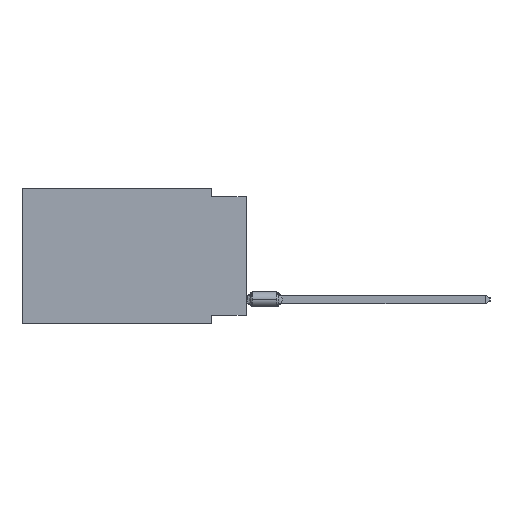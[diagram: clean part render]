
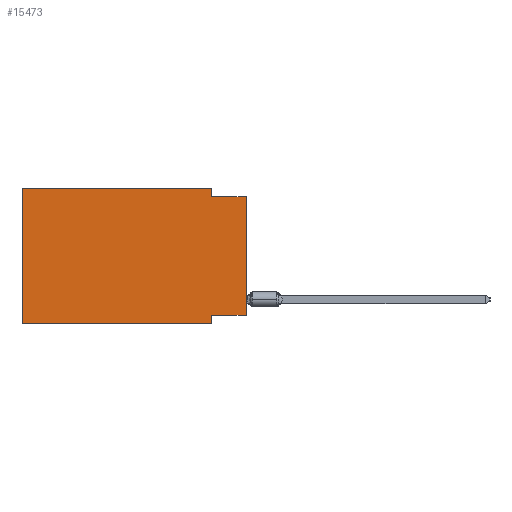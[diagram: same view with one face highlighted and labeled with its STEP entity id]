
A CAD part, left-side view. The second image highlights one B-rep face of the part: STEP entity #15473.
In plain terms, the highlighted planar face has unit normal (-1, 0, 0).
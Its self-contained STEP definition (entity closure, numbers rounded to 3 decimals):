
#1035 = DIRECTION ( 'NONE',  ( 0., -1., 0. ) ) ;
#1457 = CARTESIAN_POINT ( 'NONE',  ( 0., 0., -9.271 ) ) ;
#1651 = VECTOR ( 'NONE', #9837, 1000. ) ;
#3708 = CARTESIAN_POINT ( 'NONE',  ( 0., 2.54, 0. ) ) ;
#3875 = CARTESIAN_POINT ( 'NONE',  ( 0., 0., -9.271 ) ) ;
#4185 = EDGE_CURVE ( 'NONE', #43685, #35259, #23246, .T. ) ;
#4319 = FACE_OUTER_BOUND ( 'NONE', #26318, .T. ) ;
#5356 = EDGE_CURVE ( 'NONE', #13402, #44287, #11194, .T. ) ;
#5426 = ORIENTED_EDGE ( 'NONE', *, *, #4185, .F. ) ;
#6379 = CARTESIAN_POINT ( 'NONE',  ( 0., 0., -0.635 ) ) ;
#7292 = CARTESIAN_POINT ( 'NONE',  ( 0., 0., -0.635 ) ) ;
#7684 = EDGE_CURVE ( 'NONE', #8545, #43685, #18270, .T. ) ;
#8232 = ORIENTED_EDGE ( 'NONE', *, *, #11466, .T. ) ;
#8545 = VERTEX_POINT ( 'NONE', #31793 ) ;
#9331 = CARTESIAN_POINT ( 'NONE',  ( 0., 16.383, -9.906 ) ) ;
#9837 = DIRECTION ( 'NONE',  ( 0., -1., 0. ) ) ;
#11177 = VECTOR ( 'NONE', #12597, 1000. ) ;
#11194 = LINE ( 'NONE', #32231, #40140 ) ;
#11239 = VECTOR ( 'NONE', #1035, 1000. ) ;
#11466 = EDGE_CURVE ( 'NONE', #13402, #20700, #35704, .T. ) ;
#11579 = CARTESIAN_POINT ( 'NONE',  ( 0., 16.383, 0. ) ) ;
#12485 = ORIENTED_EDGE ( 'NONE', *, *, #7684, .F. ) ;
#12597 = DIRECTION ( 'NONE',  ( 0., 0., 1. ) ) ;
#13402 = VERTEX_POINT ( 'NONE', #9331 ) ;
#15311 = EDGE_CURVE ( 'NONE', #38041, #29236, #24675, .T. ) ;
#15473 = ADVANCED_FACE ( 'NONE', ( #4319 ), #18426, .F. ) ;
#16829 = ORIENTED_EDGE ( 'NONE', *, *, #15311, .F. ) ;
#17326 = EDGE_CURVE ( 'NONE', #38041, #35259, #40762, .T. ) ;
#18270 = LINE ( 'NONE', #3708, #45320 ) ;
#18426 = PLANE ( 'NONE',  #26439 ) ;
#18959 = CARTESIAN_POINT ( 'NONE',  ( 0., 2.54, -9.906 ) ) ;
#19021 = CARTESIAN_POINT ( 'NONE',  ( 0., 16.383, 0. ) ) ;
#19107 = CARTESIAN_POINT ( 'NONE',  ( 0., 16.383, 0. ) ) ;
#20700 = VERTEX_POINT ( 'NONE', #29949 ) ;
#22246 = LINE ( 'NONE', #19021, #34984 ) ;
#22913 = ORIENTED_EDGE ( 'NONE', *, *, #5356, .F. ) ;
#23157 = DIRECTION ( 'NONE',  ( 0., -1., 0. ) ) ;
#23246 = LINE ( 'NONE', #6379, #1651 ) ;
#23671 = CARTESIAN_POINT ( 'NONE',  ( 0., 0., 0. ) ) ;
#24661 = ORIENTED_EDGE ( 'NONE', *, *, #17326, .T. ) ;
#24675 = LINE ( 'NONE', #3875, #37514 ) ;
#26318 = EDGE_LOOP ( 'NONE', ( #24661, #5426, #12485, #37408, #22913, #8232, #43608, #16829 ) ) ;
#26439 = AXIS2_PLACEMENT_3D ( 'NONE', #19107, #33209, #35754 ) ;
#27777 = CARTESIAN_POINT ( 'NONE',  ( 0., 2.54, -9.271 ) ) ;
#29138 = LINE ( 'NONE', #18959, #42709 ) ;
#29236 = VERTEX_POINT ( 'NONE', #27777 ) ;
#29949 = CARTESIAN_POINT ( 'NONE',  ( 0., 2.54, -9.906 ) ) ;
#31396 = EDGE_CURVE ( 'NONE', #29236, #20700, #29138, .T. ) ;
#31793 = CARTESIAN_POINT ( 'NONE',  ( 0., 2.54, 0. ) ) ;
#32231 = CARTESIAN_POINT ( 'NONE',  ( 0., 16.383, 0. ) ) ;
#33209 = DIRECTION ( 'NONE',  ( 1., 0., 0. ) ) ;
#33284 = DIRECTION ( 'NONE',  ( 0., 0., -1. ) ) ;
#34984 = VECTOR ( 'NONE', #23157, 1000. ) ;
#35259 = VERTEX_POINT ( 'NONE', #7292 ) ;
#35360 = DIRECTION ( 'NONE',  ( 0., 0., -1. ) ) ;
#35689 = DIRECTION ( 'NONE',  ( 0., 0., 1. ) ) ;
#35704 = LINE ( 'NONE', #40281, #11239 ) ;
#35754 = DIRECTION ( 'NONE',  ( 0., 0., -1. ) ) ;
#37408 = ORIENTED_EDGE ( 'NONE', *, *, #43839, .F. ) ;
#37514 = VECTOR ( 'NONE', #38757, 1000. ) ;
#38041 = VERTEX_POINT ( 'NONE', #1457 ) ;
#38757 = DIRECTION ( 'NONE',  ( 0., 1., 0. ) ) ;
#39110 = CARTESIAN_POINT ( 'NONE',  ( 0., 2.54, -0.635 ) ) ;
#40140 = VECTOR ( 'NONE', #35689, 1000. ) ;
#40281 = CARTESIAN_POINT ( 'NONE',  ( 0., 16.383, -9.906 ) ) ;
#40762 = LINE ( 'NONE', #23671, #11177 ) ;
#42709 = VECTOR ( 'NONE', #33284, 1000. ) ;
#43608 = ORIENTED_EDGE ( 'NONE', *, *, #31396, .F. ) ;
#43685 = VERTEX_POINT ( 'NONE', #39110 ) ;
#43839 = EDGE_CURVE ( 'NONE', #44287, #8545, #22246, .T. ) ;
#44287 = VERTEX_POINT ( 'NONE', #11579 ) ;
#45320 = VECTOR ( 'NONE', #35360, 1000. ) ;
